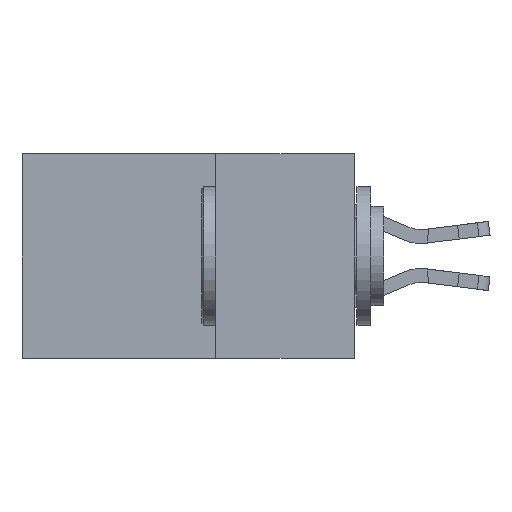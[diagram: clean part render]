
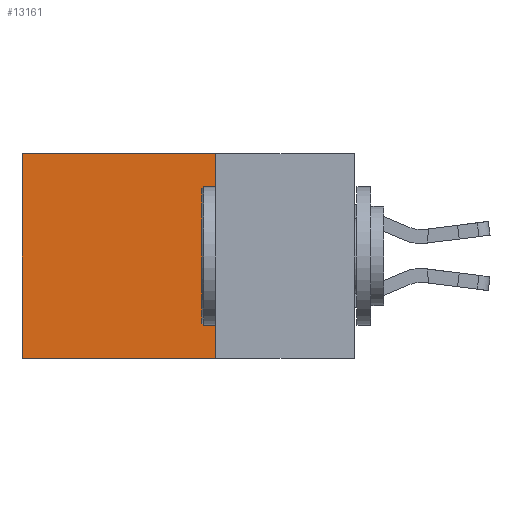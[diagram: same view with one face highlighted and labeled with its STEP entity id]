
A CAD part, left-side view. The second image highlights one B-rep face of the part: STEP entity #13161.
In plain terms, the highlighted planar face has unit normal (-1, 0, 0).
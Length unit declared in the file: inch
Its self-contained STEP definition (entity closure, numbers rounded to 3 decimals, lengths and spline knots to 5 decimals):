
#524 = LINE ( 'NONE', #4464, #8438 ) ;
#1073 = CARTESIAN_POINT ( 'NONE',  ( 0.2615, 0.6, -0.37 ) ) ;
#1426 = VERTEX_POINT ( 'NONE', #3511 ) ;
#2909 = CARTESIAN_POINT ( 'NONE',  ( 0.2615, 0.25, 0. ) ) ;
#3511 = CARTESIAN_POINT ( 'NONE',  ( 0.2615, 0.6, 0. ) ) ;
#4464 = CARTESIAN_POINT ( 'NONE',  ( 0.2615, 0.25, 0. ) ) ;
#4631 = VERTEX_POINT ( 'NONE', #5807 ) ;
#5243 = EDGE_CURVE ( 'NONE', #1426, #4631, #14123, .T. ) ;
#5631 = VECTOR ( 'NONE', #12336, 39.37008 ) ;
#5807 = CARTESIAN_POINT ( 'NONE',  ( 0.2615, 0.6, -0.37 ) ) ;
#6118 = DIRECTION ( 'NONE',  ( 0., 0., -1. ) ) ;
#7397 = FACE_OUTER_BOUND ( 'NONE', #16173, .T. ) ;
#7519 = EDGE_CURVE ( 'NONE', #16973, #9147, #11255, .T. ) ;
#7847 = DIRECTION ( 'NONE',  ( 0., 0., -1. ) ) ;
#8416 = ORIENTED_EDGE ( 'NONE', *, *, #9739, .T. ) ;
#8438 = VECTOR ( 'NONE', #13657, 39.37008 ) ;
#9004 = ORIENTED_EDGE ( 'NONE', *, *, #10067, .F. ) ;
#9147 = VERTEX_POINT ( 'NONE', #16184 ) ;
#9739 = EDGE_CURVE ( 'NONE', #16973, #1426, #524, .T. ) ;
#9884 = VECTOR ( 'NONE', #6118, 39.37008 ) ;
#10067 = EDGE_CURVE ( 'NONE', #9147, #4631, #11161, .T. ) ;
#11010 = ORIENTED_EDGE ( 'NONE', *, *, #5243, .T. ) ;
#11161 = LINE ( 'NONE', #16628, #5631 ) ;
#11255 = LINE ( 'NONE', #16547, #9884 ) ;
#11564 = ORIENTED_EDGE ( 'NONE', *, *, #7519, .F. ) ;
#11846 = DIRECTION ( 'NONE',  ( 0., 0., -1. ) ) ;
#12336 = DIRECTION ( 'NONE',  ( 0., 1., 0. ) ) ;
#12796 = CARTESIAN_POINT ( 'NONE',  ( 0.2615, 0.25, -0.37 ) ) ;
#12889 = VECTOR ( 'NONE', #11846, 39.37008 ) ;
#13161 = ADVANCED_FACE ( 'NONE', ( #7397 ), #15772, .F. ) ;
#13657 = DIRECTION ( 'NONE',  ( 0., 1., 0. ) ) ;
#14123 = LINE ( 'NONE', #1073, #12889 ) ;
#15772 = PLANE ( 'NONE',  #16872 ) ;
#16173 = EDGE_LOOP ( 'NONE', ( #11010, #9004, #11564, #8416 ) ) ;
#16184 = CARTESIAN_POINT ( 'NONE',  ( 0.2615, 0.25, -0.37 ) ) ;
#16547 = CARTESIAN_POINT ( 'NONE',  ( 0.2615, 0.25, -0.37 ) ) ;
#16628 = CARTESIAN_POINT ( 'NONE',  ( 0.2615, 0.25, -0.37 ) ) ;
#16872 = AXIS2_PLACEMENT_3D ( 'NONE', #12796, #17189, #7847 ) ;
#16973 = VERTEX_POINT ( 'NONE', #2909 ) ;
#17189 = DIRECTION ( 'NONE',  ( 1., 0., 0. ) ) ;
